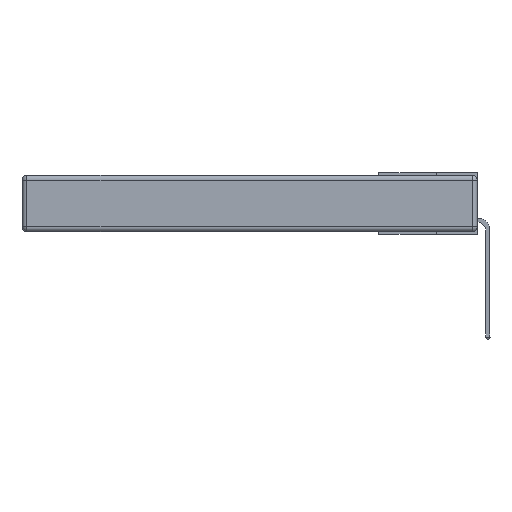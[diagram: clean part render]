
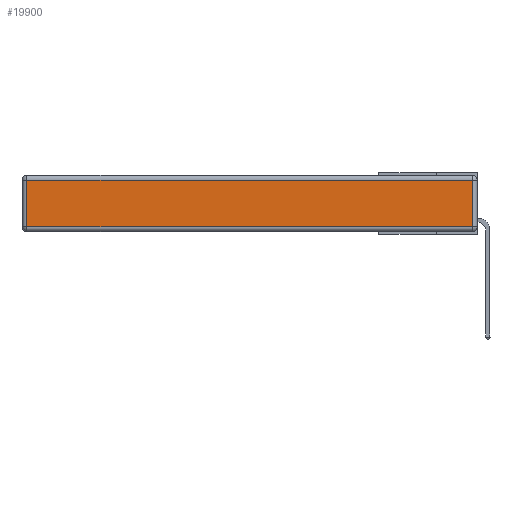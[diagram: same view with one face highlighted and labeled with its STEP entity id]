
A CAD part, left-side view. The second image highlights one B-rep face of the part: STEP entity #19900.
In plain terms, the highlighted planar face has unit normal (-1, 0, 0).
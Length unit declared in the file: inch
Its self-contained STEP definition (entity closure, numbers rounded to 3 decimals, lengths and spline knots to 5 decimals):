
#139 = CARTESIAN_POINT ( 'NONE',  ( 0., 2.72, -0.343 ) ) ;
#546 = VERTEX_POINT ( 'NONE', #20130 ) ;
#765 = DIRECTION ( 'NONE',  ( 0., 0., 1. ) ) ;
#1848 = EDGE_CURVE ( 'NONE', #546, #3964, #18835, .T. ) ;
#2295 = PLANE ( 'NONE',  #10504 ) ;
#3058 = VERTEX_POINT ( 'NONE', #20424 ) ;
#3645 = CARTESIAN_POINT ( 'NONE',  ( 0., 2.72, -0.03 ) ) ;
#3964 = VERTEX_POINT ( 'NONE', #3645 ) ;
#4394 = VERTEX_POINT ( 'NONE', #13020 ) ;
#4529 = LINE ( 'NONE', #16776, #7516 ) ;
#4790 = ORIENTED_EDGE ( 'NONE', *, *, #9981, .T. ) ;
#4829 = DIRECTION ( 'NONE',  ( 0., 0., -1. ) ) ;
#6160 = VECTOR ( 'NONE', #20111, 39.37008 ) ;
#7172 = CARTESIAN_POINT ( 'NONE',  ( 0., 0., -0.343 ) ) ;
#7516 = VECTOR ( 'NONE', #15331, 39.37008 ) ;
#8969 = LINE ( 'NONE', #139, #11730 ) ;
#9981 = EDGE_CURVE ( 'NONE', #3964, #4394, #8969, .T. ) ;
#10504 = AXIS2_PLACEMENT_3D ( 'NONE', #7172, #19734, #765 ) ;
#10732 = EDGE_CURVE ( 'NONE', #4394, #3058, #4529, .T. ) ;
#11335 = ORIENTED_EDGE ( 'NONE', *, *, #14230, .T. ) ;
#11496 = ORIENTED_EDGE ( 'NONE', *, *, #1848, .T. ) ;
#11730 = VECTOR ( 'NONE', #4829, 39.37008 ) ;
#12356 = CARTESIAN_POINT ( 'NONE',  ( 0., 2.75, -0.03 ) ) ;
#12662 = DIRECTION ( 'NONE',  ( 0., 0., 1. ) ) ;
#13020 = CARTESIAN_POINT ( 'NONE',  ( 0., 2.72, -0.313 ) ) ;
#14184 = CARTESIAN_POINT ( 'NONE',  ( 0., 0.03, -0.343 ) ) ;
#14230 = EDGE_CURVE ( 'NONE', #3058, #546, #20545, .T. ) ;
#15331 = DIRECTION ( 'NONE',  ( 0., -1., 0. ) ) ;
#16776 = CARTESIAN_POINT ( 'NONE',  ( 0., 0., -0.313 ) ) ;
#17597 = VECTOR ( 'NONE', #12662, 39.37008 ) ;
#18573 = ORIENTED_EDGE ( 'NONE', *, *, #10732, .T. ) ;
#18769 = EDGE_LOOP ( 'NONE', ( #18573, #11335, #11496, #4790 ) ) ;
#18835 = LINE ( 'NONE', #12356, #6160 ) ;
#19453 = FACE_OUTER_BOUND ( 'NONE', #18769, .T. ) ;
#19734 = DIRECTION ( 'NONE',  ( -1., 0., 0. ) ) ;
#19900 = ADVANCED_FACE ( 'NONE', ( #19453 ), #2295, .T. ) ;
#20111 = DIRECTION ( 'NONE',  ( 0., 1., 0. ) ) ;
#20130 = CARTESIAN_POINT ( 'NONE',  ( 0., 0.03, -0.03 ) ) ;
#20424 = CARTESIAN_POINT ( 'NONE',  ( 0., 0.03, -0.313 ) ) ;
#20545 = LINE ( 'NONE', #14184, #17597 ) ;
